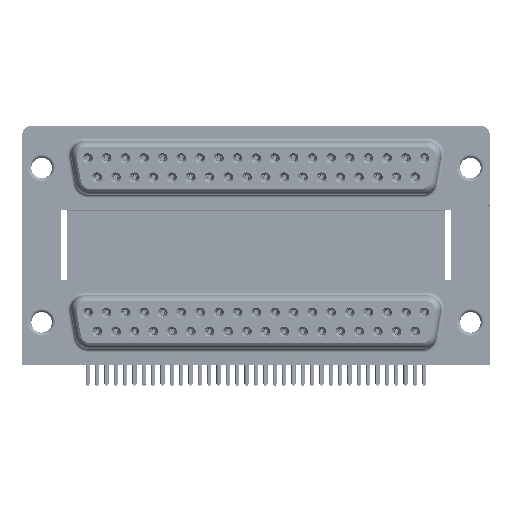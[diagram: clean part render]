
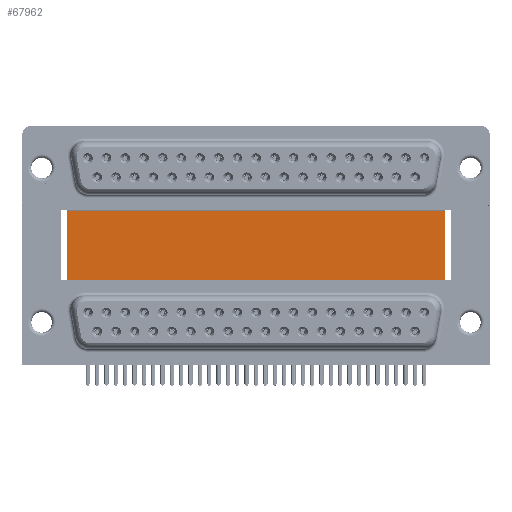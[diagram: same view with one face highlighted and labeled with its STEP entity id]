
A CAD part, top view. The second image highlights one B-rep face of the part: STEP entity #67962.
In plain terms, the highlighted planar face has unit normal (0, 0, 1).
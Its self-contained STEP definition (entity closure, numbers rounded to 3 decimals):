
#5246 = ORIENTED_EDGE ( 'NONE', *, *, #33459, .F. ) ;
#5646 = PLANE ( 'NONE',  #61428 ) ;
#11576 = DIRECTION ( 'NONE',  ( 0., -1., 0. ) ) ;
#11646 = DIRECTION ( 'NONE',  ( 0., 0., -1. ) ) ;
#11795 = CARTESIAN_POINT ( 'NONE',  ( 3.79, 16.585, -12. ) ) ;
#12625 = CARTESIAN_POINT ( 'NONE',  ( 3.79, -3.735, -12. ) ) ;
#13910 = CARTESIAN_POINT ( 'NONE',  ( 59.71, 16.585, -12. ) ) ;
#21360 = VERTEX_POINT ( 'NONE', #39759 ) ;
#24461 = VERTEX_POINT ( 'NONE', #11795 ) ;
#28145 = LINE ( 'NONE', #65480, #72065 ) ;
#28860 = VERTEX_POINT ( 'NONE', #61487 ) ;
#30573 = DIRECTION ( 'NONE',  ( 1., 0., 0. ) ) ;
#33459 = EDGE_CURVE ( 'NONE', #24461, #28860, #42640, .T. ) ;
#33827 = EDGE_LOOP ( 'NONE', ( #53154, #57096, #5246, #65787 ) ) ;
#36499 = LINE ( 'NONE', #13910, #56359 ) ;
#39759 = CARTESIAN_POINT ( 'NONE',  ( 3.79, -3.735, -12. ) ) ;
#40862 = LINE ( 'NONE', #12625, #47040 ) ;
#40992 = CARTESIAN_POINT ( 'NONE',  ( 3.79, 16.585, -12. ) ) ;
#41379 = CARTESIAN_POINT ( 'NONE',  ( 59.71, -3.735, -12. ) ) ;
#42640 = LINE ( 'NONE', #53939, #67799 ) ;
#42957 = EDGE_CURVE ( 'NONE', #24461, #21360, #28145, .T. ) ;
#46656 = FACE_OUTER_BOUND ( 'NONE', #33827, .T. ) ;
#47040 = VECTOR ( 'NONE', #47280, 1000. ) ;
#47075 = DIRECTION ( 'NONE',  ( 0., -1., 0. ) ) ;
#47280 = DIRECTION ( 'NONE',  ( 1., 0., 0. ) ) ;
#50457 = VERTEX_POINT ( 'NONE', #41379 ) ;
#53154 = ORIENTED_EDGE ( 'NONE', *, *, #60159, .T. ) ;
#53939 = CARTESIAN_POINT ( 'NONE',  ( 3.79, 16.585, -12. ) ) ;
#56359 = VECTOR ( 'NONE', #47075, 1000. ) ;
#56772 = EDGE_CURVE ( 'NONE', #28860, #50457, #36499, .T. ) ;
#57096 = ORIENTED_EDGE ( 'NONE', *, *, #56772, .F. ) ;
#57956 = DIRECTION ( 'NONE',  ( -1., 0., 0. ) ) ;
#60159 = EDGE_CURVE ( 'NONE', #21360, #50457, #40862, .T. ) ;
#61428 = AXIS2_PLACEMENT_3D ( 'NONE', #40992, #11646, #57956 ) ;
#61487 = CARTESIAN_POINT ( 'NONE',  ( 59.71, 16.585, -12. ) ) ;
#65480 = CARTESIAN_POINT ( 'NONE',  ( 3.79, 16.585, -12. ) ) ;
#65787 = ORIENTED_EDGE ( 'NONE', *, *, #42957, .T. ) ;
#67799 = VECTOR ( 'NONE', #30573, 1000. ) ;
#67962 = ADVANCED_FACE ( 'NONE', ( #46656 ), #5646, .F. ) ;
#72065 = VECTOR ( 'NONE', #11576, 1000. ) ;
